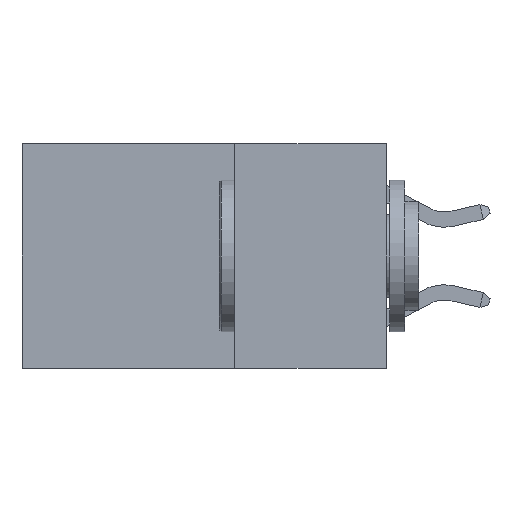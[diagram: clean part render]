
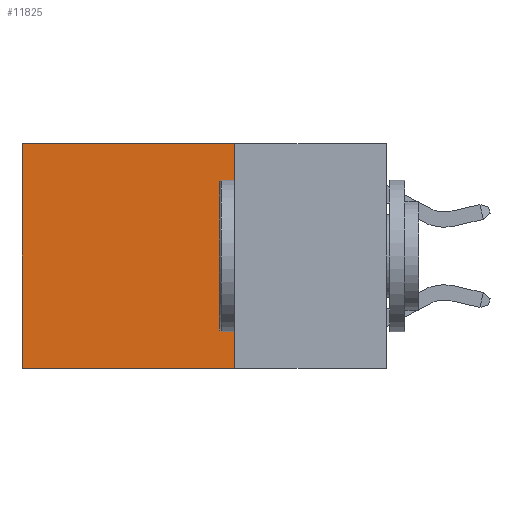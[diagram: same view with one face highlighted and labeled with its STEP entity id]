
A CAD part, left-side view. The second image highlights one B-rep face of the part: STEP entity #11825.
In plain terms, the highlighted planar face has unit normal (-1, 0, 0).
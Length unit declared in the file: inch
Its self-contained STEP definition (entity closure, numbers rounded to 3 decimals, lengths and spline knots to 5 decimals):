
#40 = VERTEX_POINT ( 'NONE', #3291 ) ;
#932 = DIRECTION ( 'NONE',  ( 1., 0., 0. ) ) ;
#1087 = DIRECTION ( 'NONE',  ( 0., 1., 0. ) ) ;
#1130 = LINE ( 'NONE', #10397, #3235 ) ;
#1382 = ORIENTED_EDGE ( 'NONE', *, *, #6349, .F. ) ;
#1519 = VERTEX_POINT ( 'NONE', #9368 ) ;
#1915 = EDGE_LOOP ( 'NONE', ( #2721, #3867, #1382, #7292 ) ) ;
#1990 = DIRECTION ( 'NONE',  ( 0., 0., -1. ) ) ;
#2424 = EDGE_CURVE ( 'NONE', #11655, #1519, #8457, .T. ) ;
#2721 = ORIENTED_EDGE ( 'NONE', *, *, #7972, .T. ) ;
#3235 = VECTOR ( 'NONE', #1990, 39.37008 ) ;
#3254 = VERTEX_POINT ( 'NONE', #7645 ) ;
#3291 = CARTESIAN_POINT ( 'NONE',  ( 0.2625, 0.25, -0.37 ) ) ;
#3850 = LINE ( 'NONE', #10275, #7183 ) ;
#3867 = ORIENTED_EDGE ( 'NONE', *, *, #6801, .F. ) ;
#4242 = LINE ( 'NONE', #9880, #6590 ) ;
#4736 = PLANE ( 'NONE',  #10767 ) ;
#4784 = VECTOR ( 'NONE', #1087, 39.37008 ) ;
#5207 = DIRECTION ( 'NONE',  ( 0., 1., 0. ) ) ;
#5400 = CARTESIAN_POINT ( 'NONE',  ( 0.2625, 0.25, 0. ) ) ;
#5591 = CARTESIAN_POINT ( 'NONE',  ( 0.2625, 0.25, 0. ) ) ;
#6349 = EDGE_CURVE ( 'NONE', #11655, #40, #1130, .T. ) ;
#6590 = VECTOR ( 'NONE', #5207, 39.37008 ) ;
#6801 = EDGE_CURVE ( 'NONE', #40, #3254, #4242, .T. ) ;
#7183 = VECTOR ( 'NONE', #11224, 39.37008 ) ;
#7292 = ORIENTED_EDGE ( 'NONE', *, *, #2424, .T. ) ;
#7645 = CARTESIAN_POINT ( 'NONE',  ( 0.2625, 0.6, -0.37 ) ) ;
#7972 = EDGE_CURVE ( 'NONE', #1519, #3254, #3850, .T. ) ;
#8457 = LINE ( 'NONE', #10348, #4784 ) ;
#9368 = CARTESIAN_POINT ( 'NONE',  ( 0.2625, 0.6, 0. ) ) ;
#9880 = CARTESIAN_POINT ( 'NONE',  ( 0.2625, 0.25, -0.37 ) ) ;
#10242 = FACE_OUTER_BOUND ( 'NONE', #1915, .T. ) ;
#10275 = CARTESIAN_POINT ( 'NONE',  ( 0.2625, 0.6, 0. ) ) ;
#10348 = CARTESIAN_POINT ( 'NONE',  ( 0.2625, 0.25, 0. ) ) ;
#10397 = CARTESIAN_POINT ( 'NONE',  ( 0.2625, 0.25, 0. ) ) ;
#10767 = AXIS2_PLACEMENT_3D ( 'NONE', #5591, #932, #11303 ) ;
#11224 = DIRECTION ( 'NONE',  ( 0., 0., -1. ) ) ;
#11303 = DIRECTION ( 'NONE',  ( 0., 0., -1. ) ) ;
#11655 = VERTEX_POINT ( 'NONE', #5400 ) ;
#11825 = ADVANCED_FACE ( 'NONE', ( #10242 ), #4736, .F. ) ;
